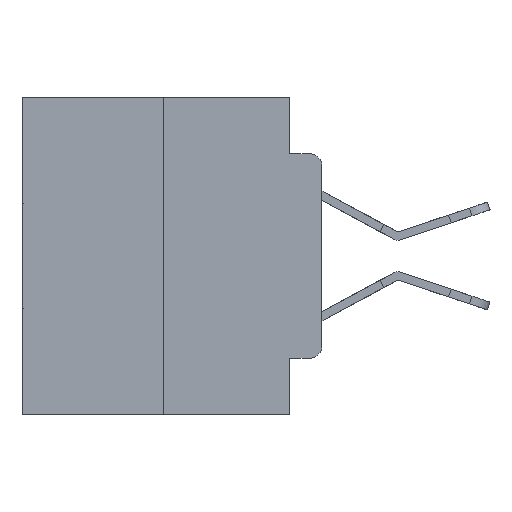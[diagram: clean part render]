
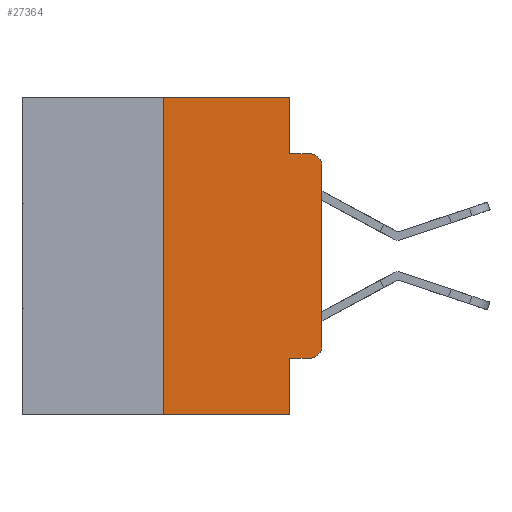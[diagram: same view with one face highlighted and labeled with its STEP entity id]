
A CAD part, left-side view. The second image highlights one B-rep face of the part: STEP entity #27364.
In plain terms, the highlighted planar face has unit normal (-1, 0, 0).
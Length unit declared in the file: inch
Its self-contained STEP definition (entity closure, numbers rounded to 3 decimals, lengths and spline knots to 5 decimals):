
#795 = ORIENTED_EDGE ( 'NONE', *, *, #12705, .F. ) ;
#1385 = DIRECTION ( 'NONE',  ( 0., 0., -1. ) ) ;
#1981 = ORIENTED_EDGE ( 'NONE', *, *, #11268, .F. ) ;
#2156 = FACE_OUTER_BOUND ( 'NONE', #11125, .T. ) ;
#3059 = VERTEX_POINT ( 'NONE', #9676 ) ;
#3410 = ORIENTED_EDGE ( 'NONE', *, *, #22354, .T. ) ;
#3538 = LINE ( 'NONE', #14900, #14794 ) ;
#3597 = AXIS2_PLACEMENT_3D ( 'NONE', #9789, #25351, #12039 ) ;
#3682 = ORIENTED_EDGE ( 'NONE', *, *, #10136, .F. ) ;
#3693 = DIRECTION ( 'NONE',  ( 0., -1., 0. ) ) ;
#4447 = EDGE_CURVE ( 'NONE', #23985, #27887, #8367, .T. ) ;
#4478 = PLANE ( 'NONE',  #24497 ) ;
#4872 = CARTESIAN_POINT ( 'NONE',  ( 0., 0.02, -0.0885 ) ) ;
#5206 = ORIENTED_EDGE ( 'NONE', *, *, #26316, .T. ) ;
#5384 = CARTESIAN_POINT ( 'NONE',  ( 0., 0.051, 0. ) ) ;
#5768 = CARTESIAN_POINT ( 'NONE',  ( 0., 0.473, -0.5 ) ) ;
#6659 = VERTEX_POINT ( 'NONE', #24917 ) ;
#6825 = CARTESIAN_POINT ( 'NONE',  ( 0., 0.473, 0. ) ) ;
#7316 = LINE ( 'NONE', #5768, #19201 ) ;
#7689 = ORIENTED_EDGE ( 'NONE', *, *, #21341, .F. ) ;
#7998 = VERTEX_POINT ( 'NONE', #21720 ) ;
#8301 = DIRECTION ( 'NONE',  ( 0., -1., 0. ) ) ;
#8367 = LINE ( 'NONE', #21655, #25420 ) ;
#8405 = CARTESIAN_POINT ( 'NONE',  ( 0., 0.051, -0.0885 ) ) ;
#9057 = DIRECTION ( 'NONE',  ( 1., 0., 0. ) ) ;
#9161 = ORIENTED_EDGE ( 'NONE', *, *, #24694, .F. ) ;
#9369 = LINE ( 'NONE', #8405, #26424 ) ;
#9373 = VECTOR ( 'NONE', #26815, 39.37008 ) ;
#9676 = CARTESIAN_POINT ( 'NONE',  ( 0., 0.051, -0.0885 ) ) ;
#9789 = CARTESIAN_POINT ( 'NONE',  ( 0., 0.02, -0.3915 ) ) ;
#10136 = EDGE_CURVE ( 'NONE', #3059, #22129, #9369, .T. ) ;
#10160 = LINE ( 'NONE', #24996, #16785 ) ;
#11125 = EDGE_LOOP ( 'NONE', ( #19192, #26344, #3682, #1981, #9161, #795, #3410, #7689, #26878, #5206 ) ) ;
#11268 = EDGE_CURVE ( 'NONE', #21748, #3059, #18027, .T. ) ;
#12039 = DIRECTION ( 'NONE',  ( 0., 0., -1. ) ) ;
#12101 = VECTOR ( 'NONE', #1385, 39.37008 ) ;
#12273 = CARTESIAN_POINT ( 'NONE',  ( 0., 0.051, -0.4115 ) ) ;
#12579 = CARTESIAN_POINT ( 'NONE',  ( 0., 0.25, 0. ) ) ;
#12705 = EDGE_CURVE ( 'NONE', #7998, #16639, #16009, .T. ) ;
#12985 = DIRECTION ( 'NONE',  ( -1., 0., 0. ) ) ;
#13471 = CARTESIAN_POINT ( 'NONE',  ( 0., 0., -0.3915 ) ) ;
#13809 = CIRCLE ( 'NONE', #17957, 0.02 ) ;
#14794 = VECTOR ( 'NONE', #3693, 39.37008 ) ;
#14857 = DIRECTION ( 'NONE',  ( 0., 0., 1. ) ) ;
#14900 = CARTESIAN_POINT ( 'NONE',  ( 0., 0.473, 0. ) ) ;
#16009 = LINE ( 'NONE', #26720, #9373 ) ;
#16639 = VERTEX_POINT ( 'NONE', #12579 ) ;
#16785 = VECTOR ( 'NONE', #20553, 39.37008 ) ;
#16927 = DIRECTION ( 'NONE',  ( 0., -1., 0. ) ) ;
#17957 = AXIS2_PLACEMENT_3D ( 'NONE', #26331, #12985, #28473 ) ;
#18027 = LINE ( 'NONE', #26037, #12101 ) ;
#19192 = ORIENTED_EDGE ( 'NONE', *, *, #4447, .T. ) ;
#19201 = VECTOR ( 'NONE', #16927, 39.37008 ) ;
#19414 = VECTOR ( 'NONE', #8301, 39.37008 ) ;
#19895 = CIRCLE ( 'NONE', #3597, 0.02 ) ;
#20091 = LINE ( 'NONE', #12273, #19414 ) ;
#20212 = VERTEX_POINT ( 'NONE', #21113 ) ;
#20553 = DIRECTION ( 'NONE',  ( 0., 0., -1. ) ) ;
#21113 = CARTESIAN_POINT ( 'NONE',  ( 0., 0.051, -0.4115 ) ) ;
#21148 = CARTESIAN_POINT ( 'NONE',  ( 0., 0.051, -0.5 ) ) ;
#21341 = EDGE_CURVE ( 'NONE', #20212, #21505, #10160, .T. ) ;
#21505 = VERTEX_POINT ( 'NONE', #21148 ) ;
#21655 = CARTESIAN_POINT ( 'NONE',  ( 0., 0., 0. ) ) ;
#21720 = CARTESIAN_POINT ( 'NONE',  ( 0., 0.25, -0.5 ) ) ;
#21748 = VERTEX_POINT ( 'NONE', #5384 ) ;
#21875 = DIRECTION ( 'NONE',  ( 0., -1., 0. ) ) ;
#22129 = VERTEX_POINT ( 'NONE', #4872 ) ;
#22354 = EDGE_CURVE ( 'NONE', #7998, #21505, #7316, .T. ) ;
#22872 = CARTESIAN_POINT ( 'NONE',  ( 0., 0., -0.1085 ) ) ;
#23985 = VERTEX_POINT ( 'NONE', #13471 ) ;
#24497 = AXIS2_PLACEMENT_3D ( 'NONE', #6825, #9057, #24649 ) ;
#24649 = DIRECTION ( 'NONE',  ( 0., 0., -1. ) ) ;
#24694 = EDGE_CURVE ( 'NONE', #16639, #21748, #3538, .T. ) ;
#24917 = CARTESIAN_POINT ( 'NONE',  ( 0., 0.02, -0.4115 ) ) ;
#24996 = CARTESIAN_POINT ( 'NONE',  ( 0., 0.051, 0. ) ) ;
#25351 = DIRECTION ( 'NONE',  ( -1., 0., 0. ) ) ;
#25420 = VECTOR ( 'NONE', #14857, 39.37008 ) ;
#26037 = CARTESIAN_POINT ( 'NONE',  ( 0., 0.051, 0. ) ) ;
#26316 = EDGE_CURVE ( 'NONE', #6659, #23985, #19895, .T. ) ;
#26331 = CARTESIAN_POINT ( 'NONE',  ( 0., 0.02, -0.1085 ) ) ;
#26344 = ORIENTED_EDGE ( 'NONE', *, *, #27607, .T. ) ;
#26424 = VECTOR ( 'NONE', #21875, 39.37008 ) ;
#26720 = CARTESIAN_POINT ( 'NONE',  ( 0., 0.25, 0. ) ) ;
#26815 = DIRECTION ( 'NONE',  ( 0., 0., 1. ) ) ;
#26878 = ORIENTED_EDGE ( 'NONE', *, *, #28650, .T. ) ;
#27364 = ADVANCED_FACE ( 'NONE', ( #2156 ), #4478, .F. ) ;
#27607 = EDGE_CURVE ( 'NONE', #27887, #22129, #13809, .T. ) ;
#27887 = VERTEX_POINT ( 'NONE', #22872 ) ;
#28473 = DIRECTION ( 'NONE',  ( 0., 0., -1. ) ) ;
#28650 = EDGE_CURVE ( 'NONE', #20212, #6659, #20091, .T. ) ;
